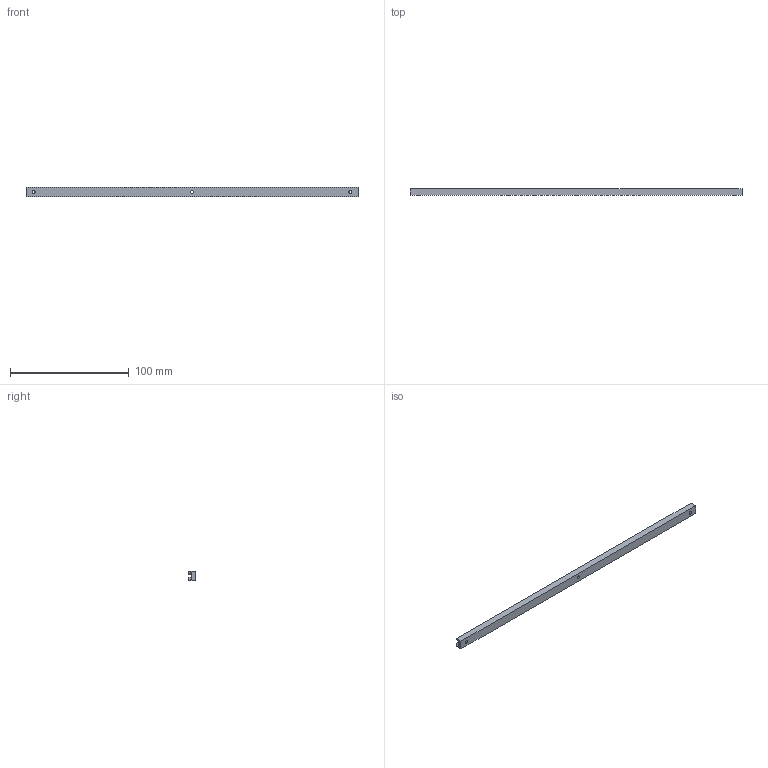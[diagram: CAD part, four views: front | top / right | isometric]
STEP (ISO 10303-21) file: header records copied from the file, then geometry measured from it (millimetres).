
FILE_DESCRIPTION (( 'STEP AP214' ), '1' );
FILE_NAME ('616-220-307.STEP', '2020-08-20T18:12:51', ( '' ), ( '' ), 'SwSTEP 2.0', 'SolidWorks 2020', '' );
FILE_SCHEMA (( 'AUTOMOTIVE_DESIGN' ));
Length unit declared in the file: inch
Products named in the file (1): 616-220-307
Bounding box: 279.4 x 5.66 x 7.92 mm (x, y, z)
Volume: 10900.7 mm3; surface area: 9011 mm2
Topology: 1 solids, 1 shells, 286 faces, 759 edges, 506 vertices
Faces by surface type: plane 180, bspline 94, cylinder 12
Entity records: 14495 total; most frequent: CARTESIAN_POINT 7934, ORIENTED_EDGE 1518, DIRECTION 993, EDGE_CURVE 759, LINE 535, VECTOR 535, VERTEX_POINT 506, EDGE_LOOP 323
